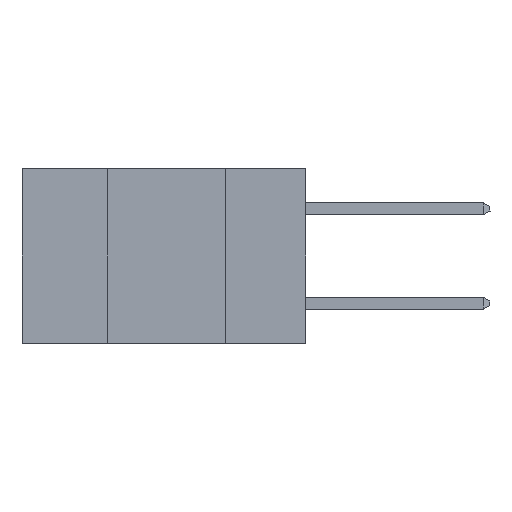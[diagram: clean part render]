
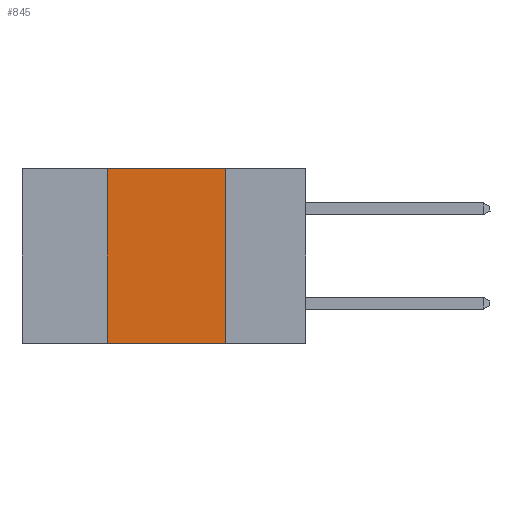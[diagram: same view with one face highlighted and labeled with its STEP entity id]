
A CAD part, left-side view. The second image highlights one B-rep face of the part: STEP entity #845.
In plain terms, the highlighted planar face has unit normal (-1, 0, 0).
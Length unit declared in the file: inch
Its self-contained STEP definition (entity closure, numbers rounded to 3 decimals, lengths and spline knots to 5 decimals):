
#365 = ORIENTED_EDGE ( 'NONE', *, *, #1549, .F. ) ;
#845 = ADVANCED_FACE ( 'NONE', ( #7997 ), #4980, .F. ) ;
#1349 = DIRECTION ( 'NONE',  ( 0., -1., 0. ) ) ;
#1357 = AXIS2_PLACEMENT_3D ( 'NONE', #8818, #5100, #2208 ) ;
#1487 = VERTEX_POINT ( 'NONE', #8973 ) ;
#1549 = EDGE_CURVE ( 'NONE', #3467, #1487, #9175, .T. ) ;
#2016 = EDGE_LOOP ( 'NONE', ( #6598, #10138, #365, #3065 ) ) ;
#2027 = CARTESIAN_POINT ( 'NONE',  ( 0., 0.17, 0. ) ) ;
#2203 = CARTESIAN_POINT ( 'NONE',  ( 0., 0.6, -0.37 ) ) ;
#2208 = DIRECTION ( 'NONE',  ( 0., 0., -1. ) ) ;
#2384 = EDGE_CURVE ( 'NONE', #8068, #10244, #4321, .T. ) ;
#2614 = CARTESIAN_POINT ( 'NONE',  ( 0., 0.42, -0.37 ) ) ;
#3065 = ORIENTED_EDGE ( 'NONE', *, *, #9185, .T. ) ;
#3467 = VERTEX_POINT ( 'NONE', #2614 ) ;
#4321 = LINE ( 'NONE', #10627, #7827 ) ;
#4499 = VECTOR ( 'NONE', #1349, 39.37008 ) ;
#4675 = CARTESIAN_POINT ( 'NONE',  ( 0., 0.42, 0. ) ) ;
#4980 = PLANE ( 'NONE',  #1357 ) ;
#5003 = DIRECTION ( 'NONE',  ( 0., 0., -1. ) ) ;
#5100 = DIRECTION ( 'NONE',  ( 1., 0., 0. ) ) ;
#5394 = CARTESIAN_POINT ( 'NONE',  ( 0., 0.17, -0.37 ) ) ;
#6535 = DIRECTION ( 'NONE',  ( 0., -1., 0. ) ) ;
#6598 = ORIENTED_EDGE ( 'NONE', *, *, #2384, .F. ) ;
#6919 = VECTOR ( 'NONE', #6535, 39.37008 ) ;
#6991 = EDGE_CURVE ( 'NONE', #1487, #8068, #9201, .T. ) ;
#7827 = VECTOR ( 'NONE', #5003, 39.37008 ) ;
#7997 = FACE_OUTER_BOUND ( 'NONE', #2016, .T. ) ;
#8068 = VERTEX_POINT ( 'NONE', #2027 ) ;
#8818 = CARTESIAN_POINT ( 'NONE',  ( 0., 0.6, 0. ) ) ;
#8860 = VECTOR ( 'NONE', #10151, 39.37008 ) ;
#8973 = CARTESIAN_POINT ( 'NONE',  ( 0., 0.42, 0. ) ) ;
#9175 = LINE ( 'NONE', #4675, #8860 ) ;
#9185 = EDGE_CURVE ( 'NONE', #3467, #10244, #9426, .T. ) ;
#9201 = LINE ( 'NONE', #9642, #4499 ) ;
#9426 = LINE ( 'NONE', #2203, #6919 ) ;
#9642 = CARTESIAN_POINT ( 'NONE',  ( 0., 0.6, 0. ) ) ;
#10138 = ORIENTED_EDGE ( 'NONE', *, *, #6991, .F. ) ;
#10151 = DIRECTION ( 'NONE',  ( 0., 0., 1. ) ) ;
#10244 = VERTEX_POINT ( 'NONE', #5394 ) ;
#10627 = CARTESIAN_POINT ( 'NONE',  ( 0., 0.17, 0. ) ) ;
